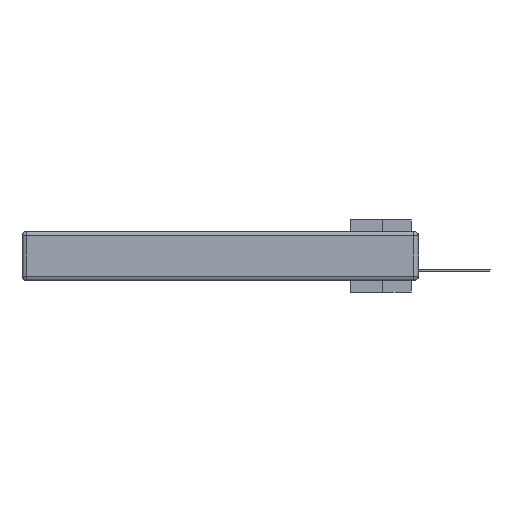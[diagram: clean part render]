
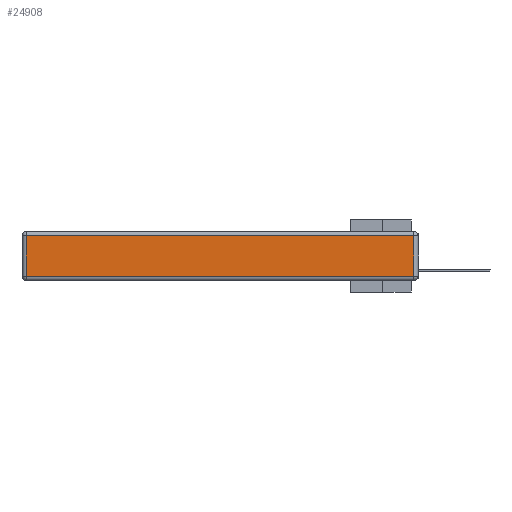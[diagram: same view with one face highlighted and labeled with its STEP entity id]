
A CAD part, left-side view. The second image highlights one B-rep face of the part: STEP entity #24908.
In plain terms, the highlighted planar face has unit normal (-1, 0, 0).
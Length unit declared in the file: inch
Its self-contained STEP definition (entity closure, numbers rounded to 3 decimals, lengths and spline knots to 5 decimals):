
#1431 = AXIS2_PLACEMENT_3D ( 'NONE', #18658, #4646, #10553 ) ;
#2683 = EDGE_CURVE ( 'NONE', #31054, #32930, #6666, .T. ) ;
#3564 = CARTESIAN_POINT ( 'NONE',  ( 0., 2.75, -0.03 ) ) ;
#3567 = ORIENTED_EDGE ( 'NONE', *, *, #34452, .T. ) ;
#4646 = DIRECTION ( 'NONE',  ( -1., 0., 0. ) ) ;
#4936 = CARTESIAN_POINT ( 'NONE',  ( 0., 0.03, -0.313 ) ) ;
#6666 = LINE ( 'NONE', #22137, #34604 ) ;
#6670 = VECTOR ( 'NONE', #26574, 39.37008 ) ;
#7489 = ORIENTED_EDGE ( 'NONE', *, *, #19569, .T. ) ;
#10553 = DIRECTION ( 'NONE',  ( 0., 0., 1. ) ) ;
#11819 = LINE ( 'NONE', #3564, #13931 ) ;
#11938 = LINE ( 'NONE', #21652, #17469 ) ;
#12376 = EDGE_LOOP ( 'NONE', ( #24038, #7489, #3567, #12605 ) ) ;
#12605 = ORIENTED_EDGE ( 'NONE', *, *, #2683, .T. ) ;
#13931 = VECTOR ( 'NONE', #33404, 39.37008 ) ;
#17416 = VERTEX_POINT ( 'NONE', #4936 ) ;
#17469 = VECTOR ( 'NONE', #29641, 39.37008 ) ;
#18658 = CARTESIAN_POINT ( 'NONE',  ( 0., 0., -0.343 ) ) ;
#19569 = EDGE_CURVE ( 'NONE', #17416, #21178, #11938, .T. ) ;
#20603 = CARTESIAN_POINT ( 'NONE',  ( 0., 0.03, -0.03 ) ) ;
#21178 = VERTEX_POINT ( 'NONE', #20603 ) ;
#21652 = CARTESIAN_POINT ( 'NONE',  ( 0., 0.03, -0.343 ) ) ;
#22137 = CARTESIAN_POINT ( 'NONE',  ( 0., 2.72, -0.343 ) ) ;
#23247 = LINE ( 'NONE', #26343, #6670 ) ;
#24038 = ORIENTED_EDGE ( 'NONE', *, *, #24968, .T. ) ;
#24908 = ADVANCED_FACE ( 'NONE', ( #26185 ), #34440, .T. ) ;
#24968 = EDGE_CURVE ( 'NONE', #32930, #17416, #23247, .T. ) ;
#26185 = FACE_OUTER_BOUND ( 'NONE', #12376, .T. ) ;
#26343 = CARTESIAN_POINT ( 'NONE',  ( 0., 0., -0.313 ) ) ;
#26574 = DIRECTION ( 'NONE',  ( 0., -1., 0. ) ) ;
#29641 = DIRECTION ( 'NONE',  ( 0., 0., 1. ) ) ;
#31054 = VERTEX_POINT ( 'NONE', #33055 ) ;
#31676 = CARTESIAN_POINT ( 'NONE',  ( 0., 2.72, -0.313 ) ) ;
#32379 = DIRECTION ( 'NONE',  ( 0., 0., -1. ) ) ;
#32930 = VERTEX_POINT ( 'NONE', #31676 ) ;
#33055 = CARTESIAN_POINT ( 'NONE',  ( 0., 2.72, -0.03 ) ) ;
#33404 = DIRECTION ( 'NONE',  ( 0., 1., 0. ) ) ;
#34440 = PLANE ( 'NONE',  #1431 ) ;
#34452 = EDGE_CURVE ( 'NONE', #21178, #31054, #11819, .T. ) ;
#34604 = VECTOR ( 'NONE', #32379, 39.37008 ) ;
